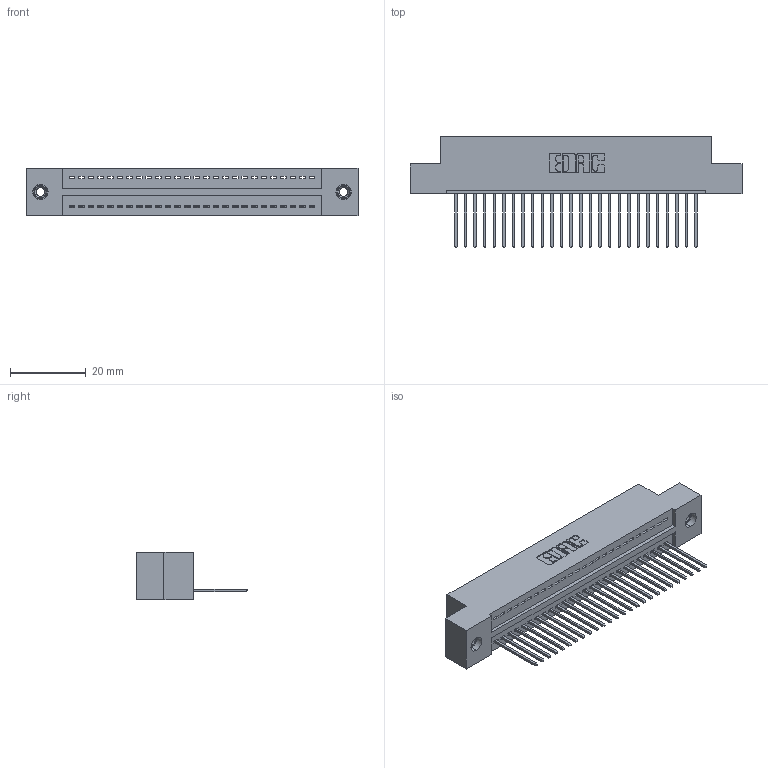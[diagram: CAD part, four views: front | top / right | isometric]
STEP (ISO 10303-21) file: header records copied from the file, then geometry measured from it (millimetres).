
FILE_DESCRIPTION (( 'STEP AP203' ), '1' );
FILE_NAME ('325-026-540-108.STEP', '2020-02-24T18:21:23', ( '' ), ( '' ), 'SwSTEP 2.0', 'SolidWorks 2016', '' );
FILE_SCHEMA (( 'CONFIG_CONTROL_DESIGN' ));
Length unit declared in the file: inch
Products named in the file (4): 325-026-540-108; 325-292-001_325-293-140; 325 Part_TI; 345-250-001_345-250-003-102
Assembly tree (29 placements, depth 2):
  325-026-540-108
    325 Part_TI
    325-292-001_325-293-140  x26
    345-250-001_345-250-003-102  x2
Bounding box: 87.76 x 29.46 x 12.45 mm (x, y, z)
Volume: 11043.7 mm3; surface area: 12069.7 mm2
Topology: 29 solids, 29 shells, 1682 faces, 5023 edges, 3306 vertices
Faces by surface type: plane 1194, cylinder 472, cone 12, torus 4
Entity records: 19168 total; most frequent: CARTESIAN_POINT 3291, ORIENTED_EDGE 3246, DIRECTION 2841, EDGE_CURVE 1623, VECTOR 1475, LINE 1475, VERTEX_POINT 1076, AXIS2_PLACEMENT_3D 683
